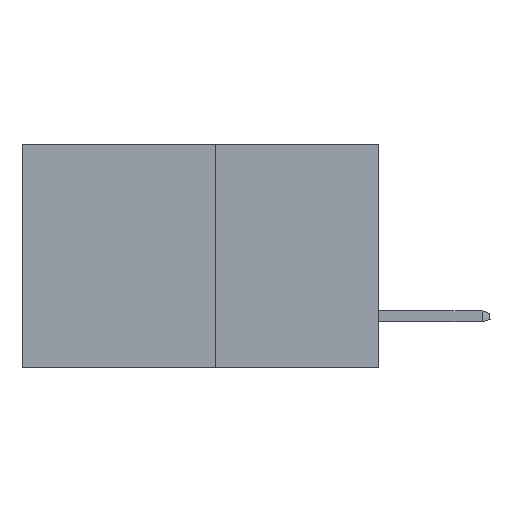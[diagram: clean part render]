
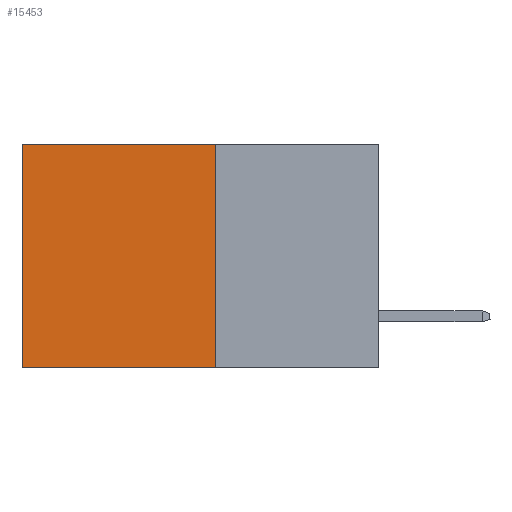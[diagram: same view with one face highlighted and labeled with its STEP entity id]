
A CAD part, left-side view. The second image highlights one B-rep face of the part: STEP entity #15453.
In plain terms, the highlighted planar face has unit normal (-1, 0, 0).
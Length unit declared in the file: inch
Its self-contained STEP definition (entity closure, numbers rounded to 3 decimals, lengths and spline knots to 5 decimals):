
#123 = PLANE ( 'NONE',  #16523 ) ;
#579 = ORIENTED_EDGE ( 'NONE', *, *, #9633, .T. ) ;
#1140 = DIRECTION ( 'NONE',  ( 0., 0., -1. ) ) ;
#1271 = CARTESIAN_POINT ( 'NONE',  ( 0.277, 0.27, -0.37 ) ) ;
#2678 = EDGE_CURVE ( 'NONE', #6093, #9062, #9195, .T. ) ;
#3127 = VECTOR ( 'NONE', #16697, 39.37008 ) ;
#4639 = LINE ( 'NONE', #1271, #13010 ) ;
#4811 = DIRECTION ( 'NONE',  ( 0., 0., -1. ) ) ;
#4974 = EDGE_CURVE ( 'NONE', #17578, #14076, #4639, .T. ) ;
#5250 = DIRECTION ( 'NONE',  ( 1., 0., 0. ) ) ;
#6093 = VERTEX_POINT ( 'NONE', #10048 ) ;
#7156 = ORIENTED_EDGE ( 'NONE', *, *, #2678, .T. ) ;
#9062 = VERTEX_POINT ( 'NONE', #10826 ) ;
#9195 = LINE ( 'NONE', #17576, #21113 ) ;
#9633 = EDGE_CURVE ( 'NONE', #17578, #6093, #18616, .T. ) ;
#9913 = VECTOR ( 'NONE', #10596, 39.37008 ) ;
#10048 = CARTESIAN_POINT ( 'NONE',  ( 0.277, 0.59, 0. ) ) ;
#10275 = CARTESIAN_POINT ( 'NONE',  ( 0.277, 0.27, -0.37 ) ) ;
#10596 = DIRECTION ( 'NONE',  ( 0., 1., 0. ) ) ;
#10826 = CARTESIAN_POINT ( 'NONE',  ( 0.277, 0.59, -0.37 ) ) ;
#11459 = CARTESIAN_POINT ( 'NONE',  ( 0.277, 0.27, 0. ) ) ;
#12722 = EDGE_CURVE ( 'NONE', #14076, #9062, #20700, .T. ) ;
#13010 = VECTOR ( 'NONE', #1140, 39.37008 ) ;
#13185 = CARTESIAN_POINT ( 'NONE',  ( 0.277, 0.27, -0.37 ) ) ;
#13854 = FACE_OUTER_BOUND ( 'NONE', #19978, .T. ) ;
#14076 = VERTEX_POINT ( 'NONE', #13185 ) ;
#15137 = CARTESIAN_POINT ( 'NONE',  ( 0.277, 0.27, -0.37 ) ) ;
#15453 = ADVANCED_FACE ( 'NONE', ( #13854 ), #123, .F. ) ;
#16523 = AXIS2_PLACEMENT_3D ( 'NONE', #10275, #5250, #16892 ) ;
#16697 = DIRECTION ( 'NONE',  ( 0., 1., 0. ) ) ;
#16892 = DIRECTION ( 'NONE',  ( 0., 0., -1. ) ) ;
#17353 = ORIENTED_EDGE ( 'NONE', *, *, #12722, .F. ) ;
#17576 = CARTESIAN_POINT ( 'NONE',  ( 0.277, 0.59, -0.37 ) ) ;
#17578 = VERTEX_POINT ( 'NONE', #11459 ) ;
#18616 = LINE ( 'NONE', #18766, #9913 ) ;
#18766 = CARTESIAN_POINT ( 'NONE',  ( 0.277, 0.27, 0. ) ) ;
#18937 = ORIENTED_EDGE ( 'NONE', *, *, #4974, .F. ) ;
#19978 = EDGE_LOOP ( 'NONE', ( #7156, #17353, #18937, #579 ) ) ;
#20700 = LINE ( 'NONE', #15137, #3127 ) ;
#21113 = VECTOR ( 'NONE', #4811, 39.37008 ) ;
